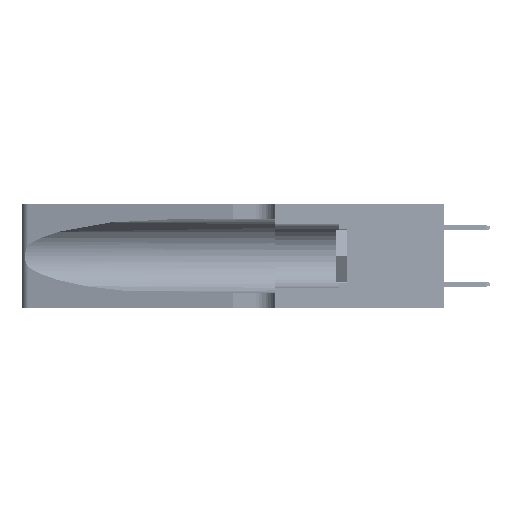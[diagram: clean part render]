
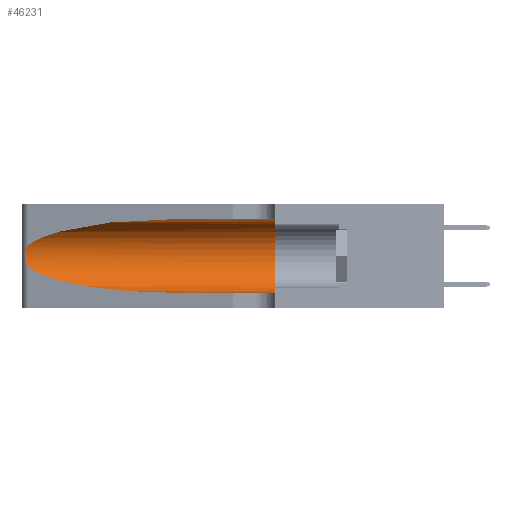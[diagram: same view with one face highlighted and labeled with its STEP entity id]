
A CAD part, left-side view. The second image highlights one B-rep face of the part: STEP entity #46231.
In plain terms, the highlighted cylindrical face has radius 3.308 mm (diameter 6.617 mm), a partial arc.
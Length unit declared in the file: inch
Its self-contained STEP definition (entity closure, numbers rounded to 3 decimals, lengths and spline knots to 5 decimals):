
#54 = CARTESIAN_POINT ( 'NONE',  ( 0.2373, 1.15595, 0.28018 ) ) ;
#874 = DIRECTION ( 'NONE',  ( 0., 0., 1. ) ) ;
#2319 = EDGE_CURVE ( 'NONE', #29454, #47307, #12718, .T. ) ;
#2685 = ORIENTED_EDGE ( 'NONE', *, *, #24373, .T. ) ;
#2883 = CARTESIAN_POINT ( 'NONE',  ( 0.25555, 1.22993, 0.14849 ) ) ;
#3525 = CARTESIAN_POINT ( 'NONE',  ( 0.26075, 1.23896, 0.178 ) ) ;
#4914 = B_SPLINE_CURVE_WITH_KNOTS ( 'NONE', 3,
 ( #29460, #6846, #29780, #36850, #18387, #22316, #14424, #3525, #29942, #18225, #25470, #41304, #2883, #33235 ),
 .UNSPECIFIED., .F., .F.,
 ( 4, 2, 2, 2, 2, 2, 4 ),
 ( 0., 0.00027, 0.00053, 0.00107, 0.0016, 0.00187, 0.00214 ),
 .UNSPECIFIED. ) ;
#5028 = DIRECTION ( 'NONE',  ( 0., -1., 0. ) ) ;
#5743 = DIRECTION ( 'NONE',  ( 0., -1., 0. ) ) ;
#5881 = CARTESIAN_POINT ( 'NONE',  ( 0.25487, 1.22718, 0.14631 ) ) ;
#6846 = CARTESIAN_POINT ( 'NONE',  ( 0.25555, 1.22994, 0.2215 ) ) ;
#8157 = CARTESIAN_POINT ( 'NONE',  ( 0.1305, 0.35, 0.185 ) ) ;
#9905 = EDGE_CURVE ( 'NONE', #10132, #47020, #14270, .T. ) ;
#10132 = VERTEX_POINT ( 'NONE', #44476 ) ;
#10240 = ORIENTED_EDGE ( 'NONE', *, *, #2319, .F. ) ;
#12550 = CARTESIAN_POINT ( 'NONE',  ( 0.1305, 1.61858, 0.185 ) ) ;
#12718 = LINE ( 'NONE', #12963, #34525 ) ;
#12963 = CARTESIAN_POINT ( 'NONE',  ( 0.1305, 1.61858, 0.31525 ) ) ;
#13682 = ORIENTED_EDGE ( 'NONE', *, *, #9905, .T. ) ;
#14270 = LINE ( 'NONE', #38908, #36088 ) ;
#14424 = CARTESIAN_POINT ( 'NONE',  ( 0.26075, 1.23896, 0.19203 ) ) ;
#15418 = ORIENTED_EDGE ( 'NONE', *, *, #24489, .T. ) ;
#16652 = CARTESIAN_POINT ( 'NONE',  ( 0.25487, 1.22718, 0.14631 ) ) ;
#16828 = AXIS2_PLACEMENT_3D ( 'NONE', #8157, #19366, #874 ) ;
#18225 = CARTESIAN_POINT ( 'NONE',  ( 0.25856, 1.23593, 0.16098 ) ) ;
#18387 = CARTESIAN_POINT ( 'NONE',  ( 0.25854, 1.2359, 0.20912 ) ) ;
#18514 = VERTEX_POINT ( 'NONE', #5881 ) ;
#18716 = CARTESIAN_POINT ( 'NONE',  ( 0.25487, 1.22718, 0.22369 ) ) ;
#19366 = DIRECTION ( 'NONE',  ( 0., 1., 0. ) ) ;
#20300 = CARTESIAN_POINT ( 'NONE',  ( 0.1305, 0.35, 0.31525 ) ) ;
#20999 =( BOUNDED_CURVE ( )  B_SPLINE_CURVE ( 3, ( #37651, #41955, #54, #18716 ),
 .UNSPECIFIED., .F., .F. ) 
 B_SPLINE_CURVE_WITH_KNOTS ( ( 4, 4 ),
 ( 1.5708, 2.84003 ),
 .UNSPECIFIED. ) 
 CURVE ( )  GEOMETRIC_REPRESENTATION_ITEM ( )  RATIONAL_B_SPLINE_CURVE ( ( 1., 0.87, 0.87, 1. ) ) 
 REPRESENTATION_ITEM ( '' )  );
#22316 = CARTESIAN_POINT ( 'NONE',  ( 0.26018, 1.23835, 0.19895 ) ) ;
#24373 = EDGE_CURVE ( 'NONE', #37396, #18514, #4914, .T. ) ;
#24489 = EDGE_CURVE ( 'NONE', #29454, #37396, #20999, .T. ) ;
#24713 = DIRECTION ( 'NONE',  ( 0., 0., -1. ) ) ;
#25470 = CARTESIAN_POINT ( 'NONE',  ( 0.25789, 1.23486, 0.15765 ) ) ;
#26033 = FACE_OUTER_BOUND ( 'NONE', #43810, .T. ) ;
#27250 = ORIENTED_EDGE ( 'NONE', *, *, #47327, .T. ) ;
#27884 = CARTESIAN_POINT ( 'NONE',  ( 0.2373, 1.15595, 0.08982 ) ) ;
#29454 = VERTEX_POINT ( 'NONE', #38686 ) ;
#29460 = CARTESIAN_POINT ( 'NONE',  ( 0.25487, 1.22718, 0.22369 ) ) ;
#29780 = CARTESIAN_POINT ( 'NONE',  ( 0.25639, 1.23184, 0.21858 ) ) ;
#29942 = CARTESIAN_POINT ( 'NONE',  ( 0.26017, 1.23833, 0.17102 ) ) ;
#32274 = ORIENTED_EDGE ( 'NONE', *, *, #33580, .F. ) ;
#33235 = CARTESIAN_POINT ( 'NONE',  ( 0.25487, 1.22718, 0.14631 ) ) ;
#33580 = EDGE_CURVE ( 'NONE', #47307, #47020, #36791, .T. ) ;
#34525 = VECTOR ( 'NONE', #5028, 39.37008 ) ;
#36088 = VECTOR ( 'NONE', #46185, 39.37008 ) ;
#36750 = AXIS2_PLACEMENT_3D ( 'NONE', #12550, #5743, #24713 ) ;
#36791 = CIRCLE ( 'NONE', #16828, 0.13025 ) ;
#36850 = CARTESIAN_POINT ( 'NONE',  ( 0.25787, 1.23484, 0.2124 ) ) ;
#37396 = VERTEX_POINT ( 'NONE', #37594 ) ;
#37434 = CARTESIAN_POINT ( 'NONE',  ( 0.1305, 0.35, 0.05475 ) ) ;
#37594 = CARTESIAN_POINT ( 'NONE',  ( 0.25487, 1.22718, 0.22369 ) ) ;
#37651 = CARTESIAN_POINT ( 'NONE',  ( 0.1305, 0.72297, 0.31525 ) ) ;
#38686 = CARTESIAN_POINT ( 'NONE',  ( 0.1305, 0.72297, 0.31525 ) ) ;
#38908 = CARTESIAN_POINT ( 'NONE',  ( 0.1305, 1.61858, 0.05475 ) ) ;
#39238 = CARTESIAN_POINT ( 'NONE',  ( 0.18966, 0.96281, 0.05475 ) ) ;
#40182 = CYLINDRICAL_SURFACE ( 'NONE', #36750, 0.13025 ) ;
#41304 = CARTESIAN_POINT ( 'NONE',  ( 0.25639, 1.23186, 0.15144 ) ) ;
#41955 = CARTESIAN_POINT ( 'NONE',  ( 0.18966, 0.96281, 0.31525 ) ) ;
#43597 =( BOUNDED_CURVE ( )  B_SPLINE_CURVE ( 3, ( #16652, #27884, #39238, #46192 ),
 .UNSPECIFIED., .F., .F. ) 
 B_SPLINE_CURVE_WITH_KNOTS ( ( 4, 4 ),
 ( 3.44316, 4.71239 ),
 .UNSPECIFIED. ) 
 CURVE ( )  GEOMETRIC_REPRESENTATION_ITEM ( )  RATIONAL_B_SPLINE_CURVE ( ( 1., 0.87, 0.87, 1. ) ) 
 REPRESENTATION_ITEM ( '' )  );
#43810 = EDGE_LOOP ( 'NONE', ( #15418, #2685, #27250, #13682, #32274, #10240 ) ) ;
#44476 = CARTESIAN_POINT ( 'NONE',  ( 0.1305, 0.72297, 0.05475 ) ) ;
#46185 = DIRECTION ( 'NONE',  ( 0., -1., 0. ) ) ;
#46192 = CARTESIAN_POINT ( 'NONE',  ( 0.1305, 0.72297, 0.05475 ) ) ;
#46231 = ADVANCED_FACE ( 'NONE', ( #26033 ), #40182, .F. ) ;
#47020 = VERTEX_POINT ( 'NONE', #37434 ) ;
#47307 = VERTEX_POINT ( 'NONE', #20300 ) ;
#47327 = EDGE_CURVE ( 'NONE', #18514, #10132, #43597, .T. ) ;
